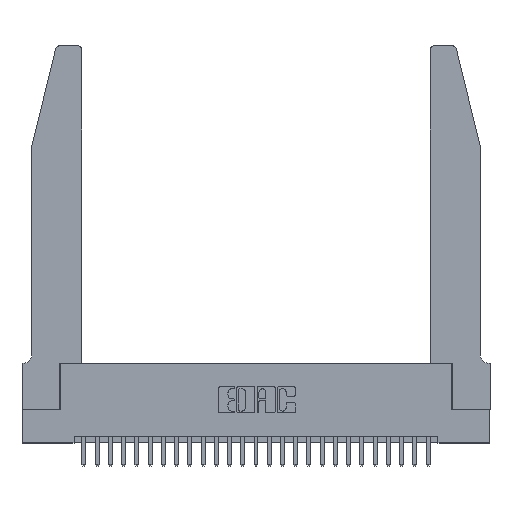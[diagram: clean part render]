
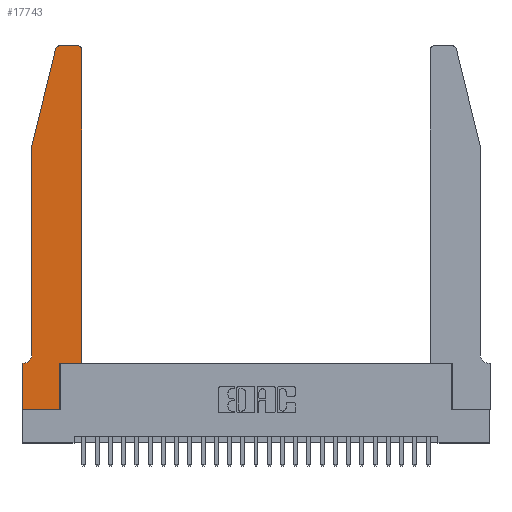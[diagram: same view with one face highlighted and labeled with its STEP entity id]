
A CAD part, top view. The second image highlights one B-rep face of the part: STEP entity #17743.
In plain terms, the highlighted planar face has unit normal (0, 0, 1).
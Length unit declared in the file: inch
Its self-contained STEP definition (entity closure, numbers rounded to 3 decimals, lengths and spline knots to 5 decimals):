
#89 = CARTESIAN_POINT ( 'NONE',  ( 0.2865, 0., 0.37 ) ) ;
#92 = VERTEX_POINT ( 'NONE', #12626 ) ;
#165 = ORIENTED_EDGE ( 'NONE', *, *, #3372, .T. ) ;
#593 = EDGE_CURVE ( 'NONE', #21878, #4587, #4120, .T. ) ;
#882 = VECTOR ( 'NONE', #14624, 39.37008 ) ;
#1402 = DIRECTION ( 'NONE',  ( 0., 1., 0. ) ) ;
#1555 = VERTEX_POINT ( 'NONE', #11207 ) ;
#1709 = EDGE_CURVE ( 'NONE', #3504, #21878, #23766, .T. ) ;
#2311 = ORIENTED_EDGE ( 'NONE', *, *, #5208, .T. ) ;
#2857 = LINE ( 'NONE', #14974, #13873 ) ;
#2866 = ORIENTED_EDGE ( 'NONE', *, *, #23355, .T. ) ;
#3372 = EDGE_CURVE ( 'NONE', #4587, #17043, #2857, .T. ) ;
#3504 = VERTEX_POINT ( 'NONE', #6634 ) ;
#4120 = CIRCLE ( 'NONE', #24189, 0.03 ) ;
#4138 = EDGE_CURVE ( 'NONE', #11823, #92, #4568, .T. ) ;
#4175 = DIRECTION ( 'NONE',  ( 0., 0., 1. ) ) ;
#4303 = VECTOR ( 'NONE', #1402, 39.37008 ) ;
#4452 = CARTESIAN_POINT ( 'NONE',  ( 0., 0., 0.37 ) ) ;
#4465 = CARTESIAN_POINT ( 'NONE',  ( 0.0055, 0.42, 0.37 ) ) ;
#4568 = CIRCLE ( 'NONE', #21602, 0.07 ) ;
#4587 = VERTEX_POINT ( 'NONE', #22860 ) ;
#5208 = EDGE_CURVE ( 'NONE', #24137, #24715, #9993, .T. ) ;
#5972 = VECTOR ( 'NONE', #16597, 39.37008 ) ;
#6179 = ORIENTED_EDGE ( 'NONE', *, *, #24342, .T. ) ;
#6384 = EDGE_CURVE ( 'NONE', #1555, #12149, #26096, .T. ) ;
#6574 = DIRECTION ( 'NONE',  ( 0., 1., 0. ) ) ;
#6634 = CARTESIAN_POINT ( 'NONE',  ( 0.4205, 2.75, 0.37 ) ) ;
#6666 = LINE ( 'NONE', #14356, #5972 ) ;
#6689 = DIRECTION ( 'NONE',  ( -1., 0., 0. ) ) ;
#6836 = LINE ( 'NONE', #16861, #882 ) ;
#7128 = CARTESIAN_POINT ( 'NONE',  ( 0.4505, 2.72, 0.37 ) ) ;
#8328 = VERTEX_POINT ( 'NONE', #7128 ) ;
#8523 = CARTESIAN_POINT ( 'NONE',  ( 0.284, 2.72, 0.37 ) ) ;
#8799 = CARTESIAN_POINT ( 'NONE',  ( 0.4505, 0.35, 0.37 ) ) ;
#9013 = DIRECTION ( 'NONE',  ( 1., 0., 0. ) ) ;
#9993 = LINE ( 'NONE', #11520, #12051 ) ;
#10028 = ORIENTED_EDGE ( 'NONE', *, *, #4138, .T. ) ;
#10646 = EDGE_CURVE ( 'NONE', #17043, #11823, #6836, .T. ) ;
#10840 = EDGE_CURVE ( 'NONE', #12149, #8328, #25076, .T. ) ;
#11207 = CARTESIAN_POINT ( 'NONE',  ( 0.2865, 0.35, 0.37 ) ) ;
#11520 = CARTESIAN_POINT ( 'NONE',  ( 0., 0., 0.37 ) ) ;
#11823 = VERTEX_POINT ( 'NONE', #20490 ) ;
#11927 = AXIS2_PLACEMENT_3D ( 'NONE', #12177, #27151, #14389 ) ;
#12051 = VECTOR ( 'NONE', #26432, 39.37008 ) ;
#12054 = CARTESIAN_POINT ( 'NONE',  ( 0.0755, 0.35, 0.37 ) ) ;
#12149 = VERTEX_POINT ( 'NONE', #8799 ) ;
#12177 = CARTESIAN_POINT ( 'NONE',  ( 0.4205, 2.72, 0.37 ) ) ;
#12626 = CARTESIAN_POINT ( 'NONE',  ( 0.0055, 0.35, 0.37 ) ) ;
#12962 = CARTESIAN_POINT ( 'NONE',  ( 0., 0.35, 0.37 ) ) ;
#13163 = CARTESIAN_POINT ( 'NONE',  ( 0.4505, 0.35, 0.37 ) ) ;
#13175 = CARTESIAN_POINT ( 'NONE',  ( 0.4505, 0.35, 0.37 ) ) ;
#13662 = VECTOR ( 'NONE', #6574, 39.37008 ) ;
#13873 = VECTOR ( 'NONE', #25703, 39.37008 ) ;
#14356 = CARTESIAN_POINT ( 'NONE',  ( 0., 0., 0.37 ) ) ;
#14389 = DIRECTION ( 'NONE',  ( 1., 0., 0. ) ) ;
#14604 = CARTESIAN_POINT ( 'NONE',  ( 0.2865, 0.35, 0.37 ) ) ;
#14624 = DIRECTION ( 'NONE',  ( 0., -1., 0. ) ) ;
#14709 = CIRCLE ( 'NONE', #11927, 0.03 ) ;
#14974 = CARTESIAN_POINT ( 'NONE',  ( 0.0755, 2., 0.37 ) ) ;
#15070 = CARTESIAN_POINT ( 'NONE',  ( 0.0755, 2., 0.37 ) ) ;
#15136 = PLANE ( 'NONE',  #15994 ) ;
#15338 = FACE_OUTER_BOUND ( 'NONE', #24502, .T. ) ;
#15415 = DIRECTION ( 'NONE',  ( 1., 0., 0. ) ) ;
#15464 = ORIENTED_EDGE ( 'NONE', *, *, #10840, .T. ) ;
#15587 = ORIENTED_EDGE ( 'NONE', *, *, #10646, .T. ) ;
#15994 = AXIS2_PLACEMENT_3D ( 'NONE', #17363, #4175, #19528 ) ;
#16014 = LINE ( 'NONE', #14604, #4303 ) ;
#16597 = DIRECTION ( 'NONE',  ( 1., 0., 0. ) ) ;
#16861 = CARTESIAN_POINT ( 'NONE',  ( 0.0755, 2., 0.37 ) ) ;
#17043 = VERTEX_POINT ( 'NONE', #15070 ) ;
#17185 = CARTESIAN_POINT ( 'NONE',  ( 0.284, 2.75, 0.37 ) ) ;
#17363 = CARTESIAN_POINT ( 'NONE',  ( 0., 0.35, 0.37 ) ) ;
#17685 = ORIENTED_EDGE ( 'NONE', *, *, #1709, .T. ) ;
#17743 = ADVANCED_FACE ( 'NONE', ( #15338 ), #15136, .T. ) ;
#18118 = VECTOR ( 'NONE', #26682, 39.37008 ) ;
#18162 = EDGE_CURVE ( 'NONE', #22511, #1555, #16014, .T. ) ;
#18575 = ORIENTED_EDGE ( 'NONE', *, *, #593, .T. ) ;
#18699 = DIRECTION ( 'NONE',  ( -1., 0., 0. ) ) ;
#19235 = EDGE_CURVE ( 'NONE', #24715, #22511, #6666, .T. ) ;
#19299 = DIRECTION ( 'NONE',  ( 0., 0., 1. ) ) ;
#19528 = DIRECTION ( 'NONE',  ( 1., 0., 0. ) ) ;
#19823 = DIRECTION ( 'NONE',  ( 0., 0., -1. ) ) ;
#20056 = ORIENTED_EDGE ( 'NONE', *, *, #19235, .T. ) ;
#20490 = CARTESIAN_POINT ( 'NONE',  ( 0.0755, 0.42, 0.37 ) ) ;
#20565 = VECTOR ( 'NONE', #15415, 39.37008 ) ;
#21602 = AXIS2_PLACEMENT_3D ( 'NONE', #4465, #19823, #6689 ) ;
#21623 = ORIENTED_EDGE ( 'NONE', *, *, #6384, .T. ) ;
#21878 = VERTEX_POINT ( 'NONE', #17185 ) ;
#22511 = VERTEX_POINT ( 'NONE', #89 ) ;
#22575 = LINE ( 'NONE', #12054, #27404 ) ;
#22860 = CARTESIAN_POINT ( 'NONE',  ( 0.25487, 2.72718, 0.37 ) ) ;
#23355 = EDGE_CURVE ( 'NONE', #92, #24137, #22575, .T. ) ;
#23766 = LINE ( 'NONE', #26594, #18118 ) ;
#24137 = VERTEX_POINT ( 'NONE', #12962 ) ;
#24189 = AXIS2_PLACEMENT_3D ( 'NONE', #8523, #19299, #9013 ) ;
#24342 = EDGE_CURVE ( 'NONE', #8328, #3504, #14709, .T. ) ;
#24502 = EDGE_LOOP ( 'NONE', ( #17685, #18575, #165, #15587, #10028, #2866, #2311, #20056, #24742, #21623, #15464, #6179 ) ) ;
#24715 = VERTEX_POINT ( 'NONE', #4452 ) ;
#24742 = ORIENTED_EDGE ( 'NONE', *, *, #18162, .T. ) ;
#25076 = LINE ( 'NONE', #13163, #13662 ) ;
#25703 = DIRECTION ( 'NONE',  ( -0.239, -0.971, 0. ) ) ;
#26096 = LINE ( 'NONE', #13175, #20565 ) ;
#26432 = DIRECTION ( 'NONE',  ( 0., -1., 0. ) ) ;
#26594 = CARTESIAN_POINT ( 'NONE',  ( 0.2605, 2.75, 0.37 ) ) ;
#26682 = DIRECTION ( 'NONE',  ( -1., 0., 0. ) ) ;
#27151 = DIRECTION ( 'NONE',  ( 0., 0., 1. ) ) ;
#27404 = VECTOR ( 'NONE', #18699, 39.37008 ) ;
